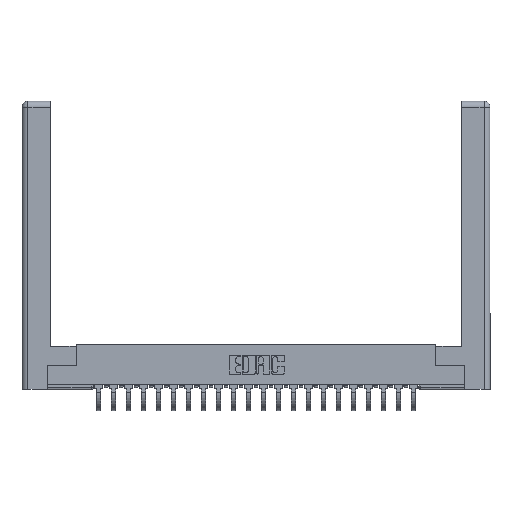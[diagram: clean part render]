
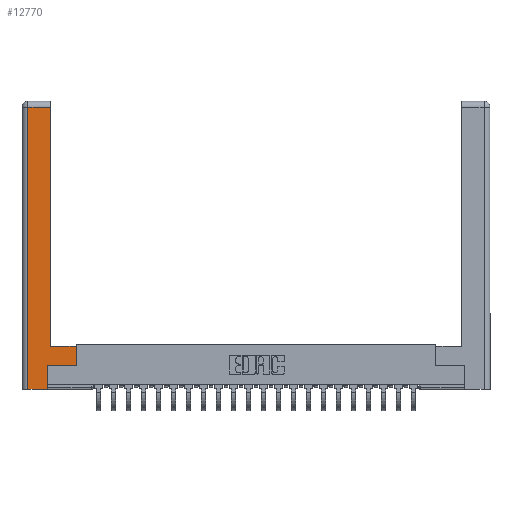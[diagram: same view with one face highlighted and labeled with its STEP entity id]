
A CAD part, top view. The second image highlights one B-rep face of the part: STEP entity #12770.
In plain terms, the highlighted planar face has unit normal (0, 0, 1).
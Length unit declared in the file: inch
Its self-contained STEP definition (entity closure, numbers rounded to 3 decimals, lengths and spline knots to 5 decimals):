
#162 = VECTOR ( 'NONE', #2415, 39.37008 ) ;
#1151 = EDGE_CURVE ( 'NONE', #2739, #1708, #17197, .T. ) ;
#1203 = DIRECTION ( 'NONE',  ( 0., 1., 0. ) ) ;
#1252 = VECTOR ( 'NONE', #1203, 39.37008 ) ;
#1291 = CARTESIAN_POINT ( 'NONE',  ( 0.0615, 2.94, 0. ) ) ;
#1557 = EDGE_CURVE ( 'NONE', #16667, #5910, #13190, .T. ) ;
#1708 = VERTEX_POINT ( 'NONE', #25639 ) ;
#2370 = CARTESIAN_POINT ( 'NONE',  ( 0.265, 0., 0. ) ) ;
#2415 = DIRECTION ( 'NONE',  ( -1., 0., 0. ) ) ;
#2557 = EDGE_CURVE ( 'NONE', #4513, #8051, #14601, .T. ) ;
#2582 = ORIENTED_EDGE ( 'NONE', *, *, #17977, .T. ) ;
#2739 = VERTEX_POINT ( 'NONE', #2370 ) ;
#3118 = CARTESIAN_POINT ( 'NONE',  ( 0.565, 0.45, 0. ) ) ;
#3140 = DIRECTION ( 'NONE',  ( -1., 0., 0. ) ) ;
#3552 = CARTESIAN_POINT ( 'NONE',  ( 0.565, 0.245, 0. ) ) ;
#4513 = VERTEX_POINT ( 'NONE', #5845 ) ;
#5387 = AXIS2_PLACEMENT_3D ( 'NONE', #11232, #25138, #13477 ) ;
#5795 = ORIENTED_EDGE ( 'NONE', *, *, #5926, .T. ) ;
#5845 = CARTESIAN_POINT ( 'NONE',  ( 0.565, 0.245, 0. ) ) ;
#5910 = VERTEX_POINT ( 'NONE', #17203 ) ;
#5926 = EDGE_CURVE ( 'NONE', #5910, #11057, #14960, .T. ) ;
#7161 = FACE_OUTER_BOUND ( 'NONE', #11583, .T. ) ;
#7593 = VECTOR ( 'NONE', #3140, 39.37008 ) ;
#7849 = CARTESIAN_POINT ( 'NONE',  ( 0.0615, 0., 0. ) ) ;
#7897 = CARTESIAN_POINT ( 'NONE',  ( 0.265, 0., 0. ) ) ;
#8051 = VERTEX_POINT ( 'NONE', #3118 ) ;
#10672 = VECTOR ( 'NONE', #20947, 39.37008 ) ;
#11057 = VERTEX_POINT ( 'NONE', #7849 ) ;
#11232 = CARTESIAN_POINT ( 'NONE',  ( 0., 0., 0. ) ) ;
#11484 = DIRECTION ( 'NONE',  ( 1., 0., 0. ) ) ;
#11583 = EDGE_LOOP ( 'NONE', ( #2582, #12511, #5795, #15246, #13919, #19886, #22487, #21806 ) ) ;
#11791 = CARTESIAN_POINT ( 'NONE',  ( 0.295, 0.45, 0. ) ) ;
#12511 = ORIENTED_EDGE ( 'NONE', *, *, #1557, .T. ) ;
#12770 = ADVANCED_FACE ( 'NONE', ( #7161 ), #17314, .F. ) ;
#12871 = EDGE_CURVE ( 'NONE', #1708, #4513, #13598, .T. ) ;
#13190 = LINE ( 'NONE', #1291, #7593 ) ;
#13477 = DIRECTION ( 'NONE',  ( -1., 0., 0. ) ) ;
#13598 = LINE ( 'NONE', #3552, #21020 ) ;
#13830 = LINE ( 'NONE', #7897, #14425 ) ;
#13919 = ORIENTED_EDGE ( 'NONE', *, *, #1151, .T. ) ;
#14221 = EDGE_CURVE ( 'NONE', #11057, #2739, #13830, .T. ) ;
#14425 = VECTOR ( 'NONE', #15951, 39.37008 ) ;
#14601 = LINE ( 'NONE', #22680, #10672 ) ;
#14960 = LINE ( 'NONE', #19315, #23534 ) ;
#15246 = ORIENTED_EDGE ( 'NONE', *, *, #14221, .T. ) ;
#15951 = DIRECTION ( 'NONE',  ( 1., 0., 0. ) ) ;
#16124 = EDGE_CURVE ( 'NONE', #8051, #17640, #20536, .T. ) ;
#16667 = VERTEX_POINT ( 'NONE', #21287 ) ;
#17197 = LINE ( 'NONE', #17320, #1252 ) ;
#17203 = CARTESIAN_POINT ( 'NONE',  ( 0.0615, 2.94, 0. ) ) ;
#17314 = PLANE ( 'NONE',  #5387 ) ;
#17315 = CARTESIAN_POINT ( 'NONE',  ( 0.295, 3., 0. ) ) ;
#17320 = CARTESIAN_POINT ( 'NONE',  ( 0.265, 0.245, 0. ) ) ;
#17640 = VERTEX_POINT ( 'NONE', #11791 ) ;
#17977 = EDGE_CURVE ( 'NONE', #17640, #16667, #23276, .T. ) ;
#19315 = CARTESIAN_POINT ( 'NONE',  ( 0.0615, 0., 0. ) ) ;
#19886 = ORIENTED_EDGE ( 'NONE', *, *, #12871, .T. ) ;
#20536 = LINE ( 'NONE', #23045, #162 ) ;
#20800 = VECTOR ( 'NONE', #23022, 39.37008 ) ;
#20947 = DIRECTION ( 'NONE',  ( 0., 1., 0. ) ) ;
#21020 = VECTOR ( 'NONE', #11484, 39.37008 ) ;
#21287 = CARTESIAN_POINT ( 'NONE',  ( 0.295, 2.94, 0. ) ) ;
#21806 = ORIENTED_EDGE ( 'NONE', *, *, #16124, .T. ) ;
#22487 = ORIENTED_EDGE ( 'NONE', *, *, #2557, .T. ) ;
#22680 = CARTESIAN_POINT ( 'NONE',  ( 0.565, 0.45, 0. ) ) ;
#23022 = DIRECTION ( 'NONE',  ( 0., 1., 0. ) ) ;
#23045 = CARTESIAN_POINT ( 'NONE',  ( 0.295, 0.45, 0. ) ) ;
#23276 = LINE ( 'NONE', #17315, #20800 ) ;
#23534 = VECTOR ( 'NONE', #25406, 39.37008 ) ;
#25138 = DIRECTION ( 'NONE',  ( 0., 0., -1. ) ) ;
#25406 = DIRECTION ( 'NONE',  ( 0., -1., 0. ) ) ;
#25639 = CARTESIAN_POINT ( 'NONE',  ( 0.265, 0.245, 0. ) ) ;
